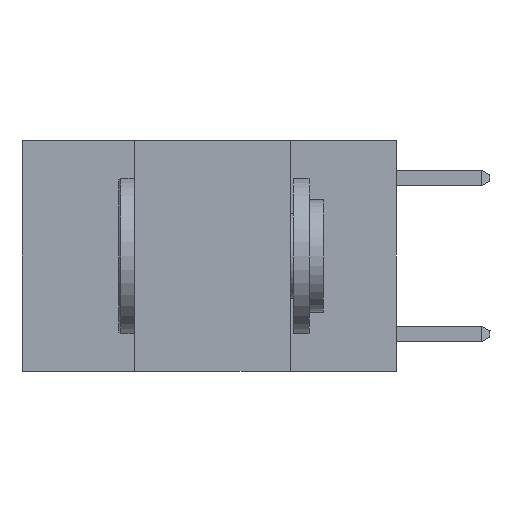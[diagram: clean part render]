
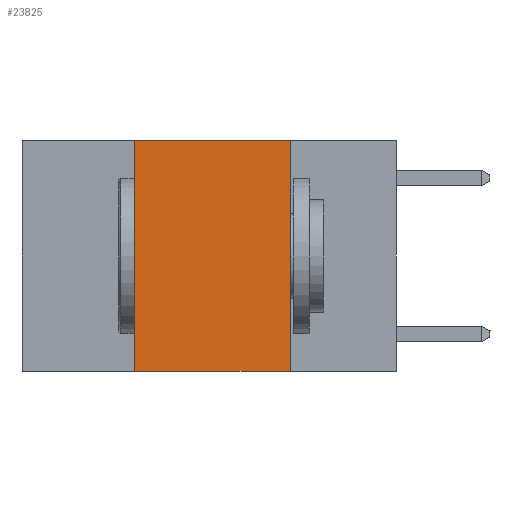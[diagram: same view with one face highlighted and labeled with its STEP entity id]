
A CAD part, left-side view. The second image highlights one B-rep face of the part: STEP entity #23825.
In plain terms, the highlighted planar face has unit normal (-1, 0, 0).
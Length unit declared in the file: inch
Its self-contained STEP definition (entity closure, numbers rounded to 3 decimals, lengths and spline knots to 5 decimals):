
#583 = CARTESIAN_POINT ( 'NONE',  ( 0., 0.6, 0. ) ) ;
#951 = VECTOR ( 'NONE', #13457, 39.37008 ) ;
#1632 = LINE ( 'NONE', #17537, #951 ) ;
#2917 = CARTESIAN_POINT ( 'NONE',  ( 0., 0.17, 0. ) ) ;
#3196 = CARTESIAN_POINT ( 'NONE',  ( 0., 0.42, 0. ) ) ;
#3620 = FACE_OUTER_BOUND ( 'NONE', #8658, .T. ) ;
#3654 = CARTESIAN_POINT ( 'NONE',  ( 0., 0.42, -0.37 ) ) ;
#3836 = CARTESIAN_POINT ( 'NONE',  ( 0., 0.17, -0.37 ) ) ;
#4953 = DIRECTION ( 'NONE',  ( 0., 0., -1. ) ) ;
#4961 = LINE ( 'NONE', #583, #20511 ) ;
#5032 = DIRECTION ( 'NONE',  ( 0., 0., -1. ) ) ;
#6832 = CARTESIAN_POINT ( 'NONE',  ( 0., 0.42, 0. ) ) ;
#7794 = LINE ( 'NONE', #3196, #17984 ) ;
#8658 = EDGE_LOOP ( 'NONE', ( #10358, #10727, #10907, #11129 ) ) ;
#9585 = VERTEX_POINT ( 'NONE', #6832 ) ;
#10358 = ORIENTED_EDGE ( 'NONE', *, *, #18893, .F. ) ;
#10727 = ORIENTED_EDGE ( 'NONE', *, *, #13320, .F. ) ;
#10907 = ORIENTED_EDGE ( 'NONE', *, *, #14865, .F. ) ;
#11129 = ORIENTED_EDGE ( 'NONE', *, *, #13476, .T. ) ;
#13006 = DIRECTION ( 'NONE',  ( 0., -1., 0. ) ) ;
#13196 = CARTESIAN_POINT ( 'NONE',  ( 0., 0.6, 0. ) ) ;
#13320 = EDGE_CURVE ( 'NONE', #9585, #23450, #4961, .T. ) ;
#13457 = DIRECTION ( 'NONE',  ( 0., -1., 0. ) ) ;
#13476 = EDGE_CURVE ( 'NONE', #21524, #20527, #1632, .T. ) ;
#14865 = EDGE_CURVE ( 'NONE', #21524, #9585, #7794, .T. ) ;
#15179 = PLANE ( 'NONE',  #23708 ) ;
#15544 = DIRECTION ( 'NONE',  ( 0., 0., 1. ) ) ;
#17260 = LINE ( 'NONE', #2917, #21250 ) ;
#17273 = DIRECTION ( 'NONE',  ( 1., 0., 0. ) ) ;
#17537 = CARTESIAN_POINT ( 'NONE',  ( 0., 0.6, -0.37 ) ) ;
#17984 = VECTOR ( 'NONE', #15544, 39.37008 ) ;
#18893 = EDGE_CURVE ( 'NONE', #23450, #20527, #17260, .T. ) ;
#20058 = CARTESIAN_POINT ( 'NONE',  ( 0., 0.17, 0. ) ) ;
#20511 = VECTOR ( 'NONE', #13006, 39.37008 ) ;
#20527 = VERTEX_POINT ( 'NONE', #3836 ) ;
#21250 = VECTOR ( 'NONE', #4953, 39.37008 ) ;
#21524 = VERTEX_POINT ( 'NONE', #3654 ) ;
#23450 = VERTEX_POINT ( 'NONE', #20058 ) ;
#23708 = AXIS2_PLACEMENT_3D ( 'NONE', #13196, #17273, #5032 ) ;
#23825 = ADVANCED_FACE ( 'NONE', ( #3620 ), #15179, .F. ) ;
